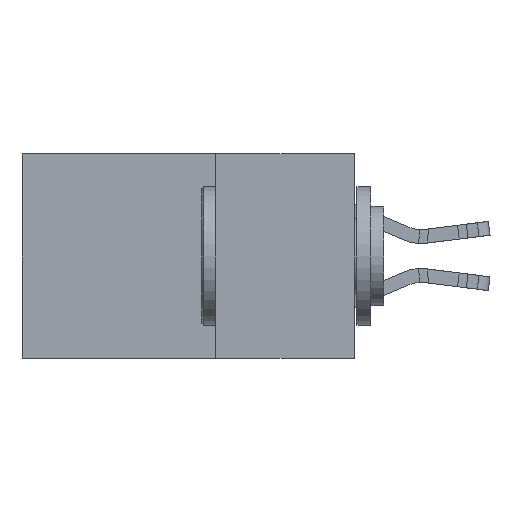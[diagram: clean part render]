
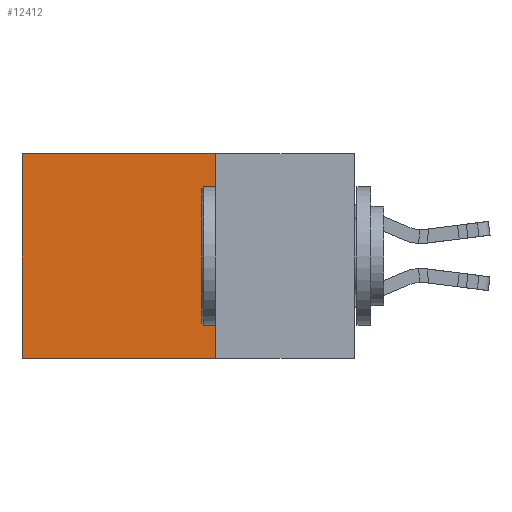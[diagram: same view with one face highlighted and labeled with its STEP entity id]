
A CAD part, left-side view. The second image highlights one B-rep face of the part: STEP entity #12412.
In plain terms, the highlighted planar face has unit normal (-1, 0, 0).
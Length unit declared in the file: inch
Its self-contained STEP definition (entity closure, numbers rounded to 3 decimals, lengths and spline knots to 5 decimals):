
#960 = DIRECTION ( 'NONE',  ( 0., 0., -1. ) ) ;
#1191 = DIRECTION ( 'NONE',  ( 0., 1., 0. ) ) ;
#1280 = DIRECTION ( 'NONE',  ( 0., 1., 0. ) ) ;
#1669 = ORIENTED_EDGE ( 'NONE', *, *, #5333, .T. ) ;
#1907 = VECTOR ( 'NONE', #1191, 39.37008 ) ;
#2149 = CARTESIAN_POINT ( 'NONE',  ( 0.2615, 0.25, 0. ) ) ;
#3616 = CARTESIAN_POINT ( 'NONE',  ( 0.2615, 0.6, -0.37 ) ) ;
#4129 = LINE ( 'NONE', #22279, #9915 ) ;
#4409 = VERTEX_POINT ( 'NONE', #19662 ) ;
#5110 = VECTOR ( 'NONE', #1280, 39.37008 ) ;
#5333 = EDGE_CURVE ( 'NONE', #4409, #15700, #18848, .T. ) ;
#6006 = AXIS2_PLACEMENT_3D ( 'NONE', #26393, #13859, #960 ) ;
#7198 = LINE ( 'NONE', #26287, #12896 ) ;
#7468 = EDGE_CURVE ( 'NONE', #15700, #20226, #7198, .T. ) ;
#9599 = PLANE ( 'NONE',  #6006 ) ;
#9768 = DIRECTION ( 'NONE',  ( 0., 0., -1. ) ) ;
#9915 = VECTOR ( 'NONE', #9768, 39.37008 ) ;
#12032 = CARTESIAN_POINT ( 'NONE',  ( 0.2615, 0.25, -0.37 ) ) ;
#12412 = ADVANCED_FACE ( 'NONE', ( #17223 ), #9599, .F. ) ;
#12896 = VECTOR ( 'NONE', #13757, 39.37008 ) ;
#13396 = EDGE_LOOP ( 'NONE', ( #21402, #17454, #22104, #1669 ) ) ;
#13757 = DIRECTION ( 'NONE',  ( 0., 0., -1. ) ) ;
#13859 = DIRECTION ( 'NONE',  ( 1., 0., 0. ) ) ;
#15700 = VERTEX_POINT ( 'NONE', #18833 ) ;
#17105 = LINE ( 'NONE', #12032, #5110 ) ;
#17223 = FACE_OUTER_BOUND ( 'NONE', #13396, .T. ) ;
#17454 = ORIENTED_EDGE ( 'NONE', *, *, #23217, .F. ) ;
#18833 = CARTESIAN_POINT ( 'NONE',  ( 0.2615, 0.6, 0. ) ) ;
#18848 = LINE ( 'NONE', #2149, #1907 ) ;
#19662 = CARTESIAN_POINT ( 'NONE',  ( 0.2615, 0.25, 0. ) ) ;
#20226 = VERTEX_POINT ( 'NONE', #3616 ) ;
#21402 = ORIENTED_EDGE ( 'NONE', *, *, #7468, .T. ) ;
#21836 = EDGE_CURVE ( 'NONE', #4409, #24684, #4129, .T. ) ;
#22104 = ORIENTED_EDGE ( 'NONE', *, *, #21836, .F. ) ;
#22225 = CARTESIAN_POINT ( 'NONE',  ( 0.2615, 0.25, -0.37 ) ) ;
#22279 = CARTESIAN_POINT ( 'NONE',  ( 0.2615, 0.25, -0.37 ) ) ;
#23217 = EDGE_CURVE ( 'NONE', #24684, #20226, #17105, .T. ) ;
#24684 = VERTEX_POINT ( 'NONE', #22225 ) ;
#26287 = CARTESIAN_POINT ( 'NONE',  ( 0.2615, 0.6, -0.37 ) ) ;
#26393 = CARTESIAN_POINT ( 'NONE',  ( 0.2615, 0.25, -0.37 ) ) ;
